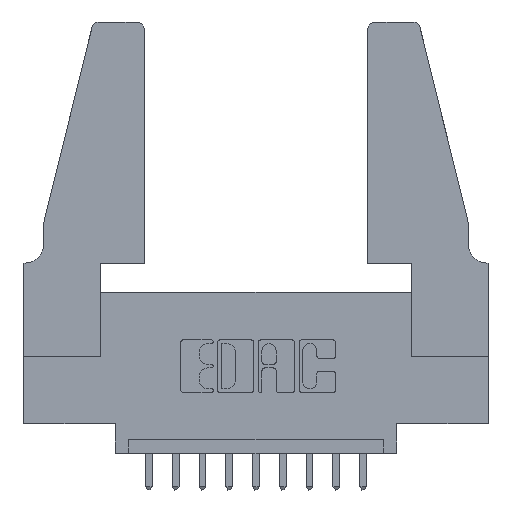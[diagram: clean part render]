
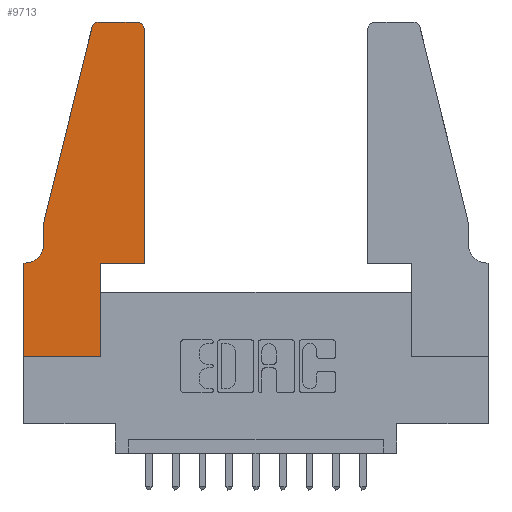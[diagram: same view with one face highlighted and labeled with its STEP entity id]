
A CAD part, top view. The second image highlights one B-rep face of the part: STEP entity #9713.
In plain terms, the highlighted planar face has unit normal (0, 0, 1).
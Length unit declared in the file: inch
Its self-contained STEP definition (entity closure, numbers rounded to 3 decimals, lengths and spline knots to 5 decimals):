
#191 = CARTESIAN_POINT ( 'NONE',  ( 0.284, 1.22, 0.37 ) ) ;
#214 = EDGE_CURVE ( 'NONE', #2952, #2103, #9898, .T. ) ;
#330 = VERTEX_POINT ( 'NONE', #4430 ) ;
#419 = VERTEX_POINT ( 'NONE', #2583 ) ;
#485 = AXIS2_PLACEMENT_3D ( 'NONE', #10737, #12684, #11824 ) ;
#544 = LINE ( 'NONE', #10210, #9332 ) ;
#814 = ORIENTED_EDGE ( 'NONE', *, *, #8453, .T. ) ;
#977 = CARTESIAN_POINT ( 'NONE',  ( 0.0755, 0.42, 0.37 ) ) ;
#1005 = CARTESIAN_POINT ( 'NONE',  ( 0.4205, 1.25, 0.37 ) ) ;
#1110 = VECTOR ( 'NONE', #7649, 39.37008 ) ;
#1180 = LINE ( 'NONE', #5809, #7837 ) ;
#1252 = DIRECTION ( 'NONE',  ( 1., 0., 0. ) ) ;
#1318 = EDGE_CURVE ( 'NONE', #9005, #12589, #3533, .T. ) ;
#1488 = ORIENTED_EDGE ( 'NONE', *, *, #10213, .T. ) ;
#2103 = VERTEX_POINT ( 'NONE', #8957 ) ;
#2204 = ORIENTED_EDGE ( 'NONE', *, *, #8612, .T. ) ;
#2224 = DIRECTION ( 'NONE',  ( -1., 0., 0. ) ) ;
#2266 = DIRECTION ( 'NONE',  ( 1., 0., 0. ) ) ;
#2583 = CARTESIAN_POINT ( 'NONE',  ( 0.0055, 0.35, 0.37 ) ) ;
#2624 = DIRECTION ( 'NONE',  ( 0., 1., 0. ) ) ;
#2766 = DIRECTION ( 'NONE',  ( -1., 0., 0. ) ) ;
#2886 = CARTESIAN_POINT ( 'NONE',  ( 0.4205, 1.22, 0.37 ) ) ;
#2913 = VECTOR ( 'NONE', #10404, 39.37008 ) ;
#2952 = VERTEX_POINT ( 'NONE', #6396 ) ;
#3293 = ORIENTED_EDGE ( 'NONE', *, *, #10946, .T. ) ;
#3451 = CIRCLE ( 'NONE', #11099, 0.03 ) ;
#3492 = LINE ( 'NONE', #6139, #12487 ) ;
#3520 = CARTESIAN_POINT ( 'NONE',  ( 0.0755, 0.5, 0.37 ) ) ;
#3533 = LINE ( 'NONE', #10993, #12525 ) ;
#3552 = AXIS2_PLACEMENT_3D ( 'NONE', #6352, #6300, #10529 ) ;
#3612 = CARTESIAN_POINT ( 'NONE',  ( 0.4505, 0.35, 0.37 ) ) ;
#4430 = CARTESIAN_POINT ( 'NONE',  ( 0.2865, 0., 0.37 ) ) ;
#4725 = CARTESIAN_POINT ( 'NONE',  ( 0.2865, 0.35, 0.37 ) ) ;
#4833 = DIRECTION ( 'NONE',  ( 1., 0., 0. ) ) ;
#5157 = CARTESIAN_POINT ( 'NONE',  ( 0., 0., 0.37 ) ) ;
#5192 = EDGE_CURVE ( 'NONE', #330, #6389, #9081, .T. ) ;
#5201 = CARTESIAN_POINT ( 'NONE',  ( 0.4505, 0.35, 0.37 ) ) ;
#5227 = CARTESIAN_POINT ( 'NONE',  ( 0.0755, 0.35, 0.37 ) ) ;
#5396 = PLANE ( 'NONE',  #485 ) ;
#5512 = ORIENTED_EDGE ( 'NONE', *, *, #5849, .T. ) ;
#5572 = ORIENTED_EDGE ( 'NONE', *, *, #12082, .T. ) ;
#5809 = CARTESIAN_POINT ( 'NONE',  ( 0.0755, 0.5, 0.37 ) ) ;
#5849 = EDGE_CURVE ( 'NONE', #419, #6724, #6939, .T. ) ;
#5879 = DIRECTION ( 'NONE',  ( 0., 0., 1. ) ) ;
#5948 = VERTEX_POINT ( 'NONE', #7438 ) ;
#6139 = CARTESIAN_POINT ( 'NONE',  ( 0.4505, 0.35, 0.37 ) ) ;
#6149 = VERTEX_POINT ( 'NONE', #3612 ) ;
#6300 = DIRECTION ( 'NONE',  ( 0., 0., -1. ) ) ;
#6352 = CARTESIAN_POINT ( 'NONE',  ( 0.0055, 0.42, 0.37 ) ) ;
#6389 = VERTEX_POINT ( 'NONE', #8765 ) ;
#6396 = CARTESIAN_POINT ( 'NONE',  ( 0.25487, 1.22718, 0.37 ) ) ;
#6503 = ORIENTED_EDGE ( 'NONE', *, *, #214, .T. ) ;
#6724 = VERTEX_POINT ( 'NONE', #6852 ) ;
#6845 = FACE_OUTER_BOUND ( 'NONE', #12959, .T. ) ;
#6852 = CARTESIAN_POINT ( 'NONE',  ( 0., 0.35, 0.37 ) ) ;
#6939 = LINE ( 'NONE', #5227, #9716 ) ;
#7438 = CARTESIAN_POINT ( 'NONE',  ( 0.4505, 1.22, 0.37 ) ) ;
#7474 = DIRECTION ( 'NONE',  ( 0., 0., 1. ) ) ;
#7484 = LINE ( 'NONE', #5157, #2913 ) ;
#7649 = DIRECTION ( 'NONE',  ( -0.239, -0.971, 0. ) ) ;
#7837 = VECTOR ( 'NONE', #7901, 39.37008 ) ;
#7901 = DIRECTION ( 'NONE',  ( 0., -1., 0. ) ) ;
#8068 = VERTEX_POINT ( 'NONE', #10370 ) ;
#8453 = EDGE_CURVE ( 'NONE', #12589, #2952, #3451, .T. ) ;
#8612 = EDGE_CURVE ( 'NONE', #6389, #6149, #10609, .T. ) ;
#8765 = CARTESIAN_POINT ( 'NONE',  ( 0.2865, 0.35, 0.37 ) ) ;
#8957 = CARTESIAN_POINT ( 'NONE',  ( 0.0755, 0.5, 0.37 ) ) ;
#9005 = VERTEX_POINT ( 'NONE', #1005 ) ;
#9081 = LINE ( 'NONE', #4725, #10859 ) ;
#9332 = VECTOR ( 'NONE', #2266, 39.37008 ) ;
#9488 = AXIS2_PLACEMENT_3D ( 'NONE', #2886, #5879, #4833 ) ;
#9579 = DIRECTION ( 'NONE',  ( 0., 1., 0. ) ) ;
#9713 = ADVANCED_FACE ( 'NONE', ( #6845 ), #5396, .T. ) ;
#9716 = VECTOR ( 'NONE', #2224, 39.37008 ) ;
#9898 = LINE ( 'NONE', #3520, #1110 ) ;
#10091 = EDGE_CURVE ( 'NONE', #5948, #9005, #13062, .T. ) ;
#10194 = ORIENTED_EDGE ( 'NONE', *, *, #10091, .T. ) ;
#10210 = CARTESIAN_POINT ( 'NONE',  ( 0., 0., 0.37 ) ) ;
#10213 = EDGE_CURVE ( 'NONE', #6724, #8068, #7484, .T. ) ;
#10370 = CARTESIAN_POINT ( 'NONE',  ( 0., 0., 0.37 ) ) ;
#10404 = DIRECTION ( 'NONE',  ( 0., -1., 0. ) ) ;
#10529 = DIRECTION ( 'NONE',  ( -1., 0., 0. ) ) ;
#10609 = LINE ( 'NONE', #5201, #12755 ) ;
#10737 = CARTESIAN_POINT ( 'NONE',  ( 0., 0.35, 0.37 ) ) ;
#10761 = ORIENTED_EDGE ( 'NONE', *, *, #13396, .T. ) ;
#10859 = VECTOR ( 'NONE', #2624, 39.37008 ) ;
#10946 = EDGE_CURVE ( 'NONE', #6149, #5948, #3492, .T. ) ;
#10993 = CARTESIAN_POINT ( 'NONE',  ( 0.2605, 1.25, 0.37 ) ) ;
#11099 = AXIS2_PLACEMENT_3D ( 'NONE', #191, #7474, #1252 ) ;
#11633 = CIRCLE ( 'NONE', #3552, 0.07 ) ;
#11824 = DIRECTION ( 'NONE',  ( 1., 0., 0. ) ) ;
#11833 = CARTESIAN_POINT ( 'NONE',  ( 0.284, 1.25, 0.37 ) ) ;
#11954 = VERTEX_POINT ( 'NONE', #977 ) ;
#12066 = ORIENTED_EDGE ( 'NONE', *, *, #1318, .T. ) ;
#12082 = EDGE_CURVE ( 'NONE', #11954, #419, #11633, .T. ) ;
#12112 = EDGE_CURVE ( 'NONE', #8068, #330, #544, .T. ) ;
#12487 = VECTOR ( 'NONE', #9579, 39.37008 ) ;
#12525 = VECTOR ( 'NONE', #2766, 39.37008 ) ;
#12589 = VERTEX_POINT ( 'NONE', #11833 ) ;
#12684 = DIRECTION ( 'NONE',  ( 0., 0., 1. ) ) ;
#12755 = VECTOR ( 'NONE', #13496, 39.37008 ) ;
#12959 = EDGE_LOOP ( 'NONE', ( #12066, #814, #6503, #10761, #5572, #5512, #1488, #13535, #13212, #2204, #3293, #10194 ) ) ;
#13062 = CIRCLE ( 'NONE', #9488, 0.03 ) ;
#13212 = ORIENTED_EDGE ( 'NONE', *, *, #5192, .T. ) ;
#13396 = EDGE_CURVE ( 'NONE', #2103, #11954, #1180, .T. ) ;
#13496 = DIRECTION ( 'NONE',  ( 1., 0., 0. ) ) ;
#13535 = ORIENTED_EDGE ( 'NONE', *, *, #12112, .T. ) ;
